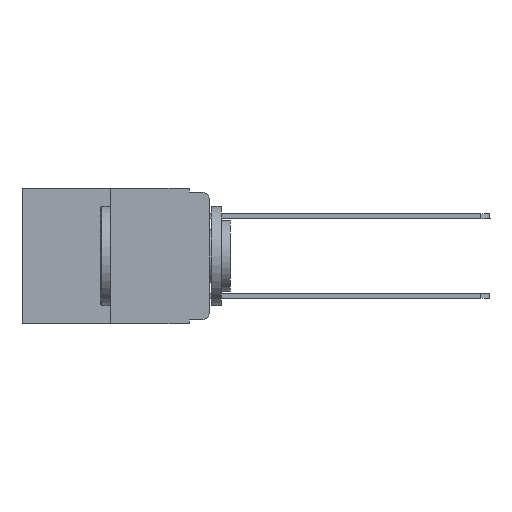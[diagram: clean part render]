
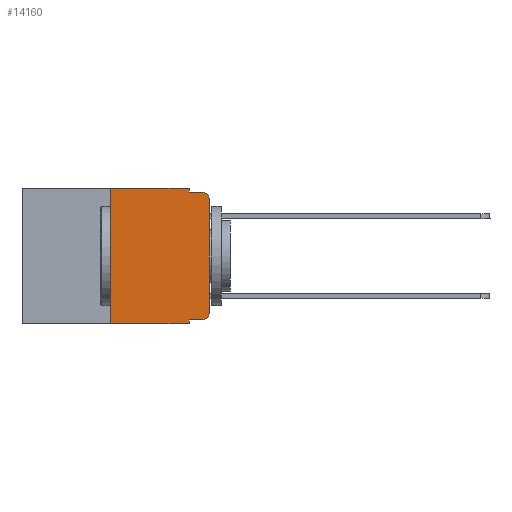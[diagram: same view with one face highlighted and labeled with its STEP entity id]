
A CAD part, left-side view. The second image highlights one B-rep face of the part: STEP entity #14160.
In plain terms, the highlighted planar face has unit normal (-1, 0, 0).
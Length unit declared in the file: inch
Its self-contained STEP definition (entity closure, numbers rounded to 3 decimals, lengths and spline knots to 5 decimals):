
#264 = ORIENTED_EDGE ( 'NONE', *, *, #11528, .F. ) ;
#637 = CARTESIAN_POINT ( 'NONE',  ( 0., 0., -0.313 ) ) ;
#831 = EDGE_CURVE ( 'NONE', #1550, #13633, #10853, .T. ) ;
#985 = ORIENTED_EDGE ( 'NONE', *, *, #14633, .T. ) ;
#1358 = VECTOR ( 'NONE', #3023, 39.37008 ) ;
#1476 = ORIENTED_EDGE ( 'NONE', *, *, #831, .T. ) ;
#1550 = VERTEX_POINT ( 'NONE', #13681 ) ;
#1883 = DIRECTION ( 'NONE',  ( 0., -1., 0. ) ) ;
#2034 = DIRECTION ( 'NONE',  ( 0., -1., 0. ) ) ;
#2084 = ORIENTED_EDGE ( 'NONE', *, *, #14444, .F. ) ;
#2121 = DIRECTION ( 'NONE',  ( 0., 0., -1. ) ) ;
#2326 = CARTESIAN_POINT ( 'NONE',  ( 0., 0.051, -0.01 ) ) ;
#2666 = ORIENTED_EDGE ( 'NONE', *, *, #13570, .T. ) ;
#2743 = VERTEX_POINT ( 'NONE', #5626 ) ;
#2754 = ORIENTED_EDGE ( 'NONE', *, *, #9873, .F. ) ;
#3009 = VECTOR ( 'NONE', #2034, 39.37008 ) ;
#3023 = DIRECTION ( 'NONE',  ( 0., -1., 0. ) ) ;
#3436 = EDGE_LOOP ( 'NONE', ( #11789, #2666, #2754, #264, #15280, #6988, #1476, #2084, #985, #13140 ) ) ;
#4528 = VECTOR ( 'NONE', #16784, 39.37008 ) ;
#4539 = DIRECTION ( 'NONE',  ( 0., 0., -1. ) ) ;
#4647 = CARTESIAN_POINT ( 'NONE',  ( 0., 0.051, -0.01 ) ) ;
#4714 = LINE ( 'NONE', #15248, #19139 ) ;
#4928 = DIRECTION ( 'NONE',  ( 1., 0., 0. ) ) ;
#5168 = AXIS2_PLACEMENT_3D ( 'NONE', #5460, #17625, #18990 ) ;
#5304 = VERTEX_POINT ( 'NONE', #14616 ) ;
#5460 = CARTESIAN_POINT ( 'NONE',  ( 0., 0.02, -0.03 ) ) ;
#5626 = CARTESIAN_POINT ( 'NONE',  ( 0., 0., -0.03 ) ) ;
#5934 = VERTEX_POINT ( 'NONE', #9478 ) ;
#6462 = CARTESIAN_POINT ( 'NONE',  ( 0., 0.473, -0.343 ) ) ;
#6988 = ORIENTED_EDGE ( 'NONE', *, *, #10908, .F. ) ;
#7076 = CARTESIAN_POINT ( 'NONE',  ( 0., 0.02, -0.333 ) ) ;
#7154 = CARTESIAN_POINT ( 'NONE',  ( 0., 0.051, 0. ) ) ;
#7509 = CARTESIAN_POINT ( 'NONE',  ( 0., 0.051, -0.343 ) ) ;
#7548 = DIRECTION ( 'NONE',  ( 0., 0., 1. ) ) ;
#7650 = AXIS2_PLACEMENT_3D ( 'NONE', #17984, #15265, #4539 ) ;
#7717 = EDGE_CURVE ( 'NONE', #13309, #2743, #10668, .T. ) ;
#8606 = AXIS2_PLACEMENT_3D ( 'NONE', #12170, #4928, #11961 ) ;
#8951 = VERTEX_POINT ( 'NONE', #13203 ) ;
#9129 = FACE_OUTER_BOUND ( 'NONE', #3436, .T. ) ;
#9478 = CARTESIAN_POINT ( 'NONE',  ( 0., 0.25, 0. ) ) ;
#9873 = EDGE_CURVE ( 'NONE', #18289, #8951, #14330, .T. ) ;
#10085 = DIRECTION ( 'NONE',  ( 0., 0., -1. ) ) ;
#10286 = LINE ( 'NONE', #7154, #15125 ) ;
#10668 = LINE ( 'NONE', #16585, #16399 ) ;
#10853 = LINE ( 'NONE', #6462, #4528 ) ;
#10908 = EDGE_CURVE ( 'NONE', #1550, #5934, #18029, .T. ) ;
#11097 = CARTESIAN_POINT ( 'NONE',  ( 0., 0.051, 0. ) ) ;
#11220 = EDGE_CURVE ( 'NONE', #5934, #15211, #19165, .T. ) ;
#11507 = CARTESIAN_POINT ( 'NONE',  ( 0., 0.473, 0. ) ) ;
#11528 = EDGE_CURVE ( 'NONE', #15211, #18289, #18580, .T. ) ;
#11789 = ORIENTED_EDGE ( 'NONE', *, *, #7717, .T. ) ;
#11961 = DIRECTION ( 'NONE',  ( 0., 0., -1. ) ) ;
#12170 = CARTESIAN_POINT ( 'NONE',  ( 0., 0.473, 0. ) ) ;
#12300 = CARTESIAN_POINT ( 'NONE',  ( 0., 0.051, 0. ) ) ;
#12868 = VECTOR ( 'NONE', #15396, 39.37008 ) ;
#13047 = VERTEX_POINT ( 'NONE', #7076 ) ;
#13123 = EDGE_CURVE ( 'NONE', #13047, #13309, #17893, .T. ) ;
#13140 = ORIENTED_EDGE ( 'NONE', *, *, #13123, .T. ) ;
#13203 = CARTESIAN_POINT ( 'NONE',  ( 0., 0.02, -0.01 ) ) ;
#13309 = VERTEX_POINT ( 'NONE', #637 ) ;
#13570 = EDGE_CURVE ( 'NONE', #2743, #8951, #16975, .T. ) ;
#13633 = VERTEX_POINT ( 'NONE', #7509 ) ;
#13681 = CARTESIAN_POINT ( 'NONE',  ( 0., 0.25, -0.343 ) ) ;
#13710 = PLANE ( 'NONE',  #8606 ) ;
#13947 = CARTESIAN_POINT ( 'NONE',  ( 0., 0.25, 0. ) ) ;
#14160 = ADVANCED_FACE ( 'NONE', ( #9129 ), #13710, .F. ) ;
#14330 = LINE ( 'NONE', #2326, #3009 ) ;
#14444 = EDGE_CURVE ( 'NONE', #5304, #13633, #10286, .T. ) ;
#14616 = CARTESIAN_POINT ( 'NONE',  ( 0., 0.051, -0.333 ) ) ;
#14633 = EDGE_CURVE ( 'NONE', #5304, #13047, #4714, .T. ) ;
#15125 = VECTOR ( 'NONE', #10085, 39.37008 ) ;
#15211 = VERTEX_POINT ( 'NONE', #12300 ) ;
#15248 = CARTESIAN_POINT ( 'NONE',  ( 0., 0.051, -0.333 ) ) ;
#15265 = DIRECTION ( 'NONE',  ( -1., 0., 0. ) ) ;
#15280 = ORIENTED_EDGE ( 'NONE', *, *, #11220, .F. ) ;
#15396 = DIRECTION ( 'NONE',  ( 0., 0., 1. ) ) ;
#16399 = VECTOR ( 'NONE', #7548, 39.37008 ) ;
#16585 = CARTESIAN_POINT ( 'NONE',  ( 0., 0., 0. ) ) ;
#16784 = DIRECTION ( 'NONE',  ( 0., -1., 0. ) ) ;
#16975 = CIRCLE ( 'NONE', #5168, 0.02 ) ;
#17625 = DIRECTION ( 'NONE',  ( -1., 0., 0. ) ) ;
#17893 = CIRCLE ( 'NONE', #7650, 0.02 ) ;
#17984 = CARTESIAN_POINT ( 'NONE',  ( 0., 0.02, -0.313 ) ) ;
#18029 = LINE ( 'NONE', #13947, #12868 ) ;
#18289 = VERTEX_POINT ( 'NONE', #4647 ) ;
#18580 = LINE ( 'NONE', #11097, #19100 ) ;
#18990 = DIRECTION ( 'NONE',  ( 0., 0., -1. ) ) ;
#19100 = VECTOR ( 'NONE', #2121, 39.37008 ) ;
#19139 = VECTOR ( 'NONE', #1883, 39.37008 ) ;
#19165 = LINE ( 'NONE', #11507, #1358 ) ;
